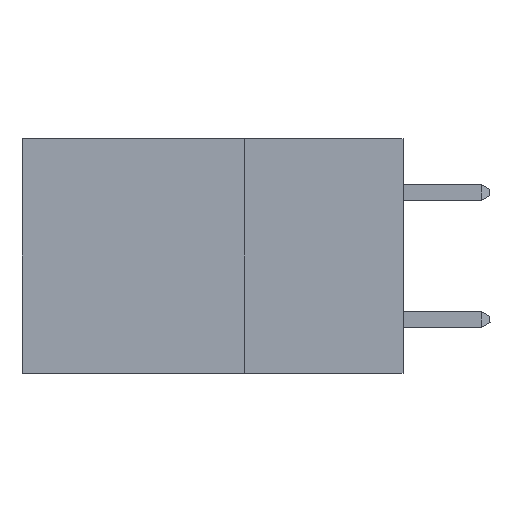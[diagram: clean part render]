
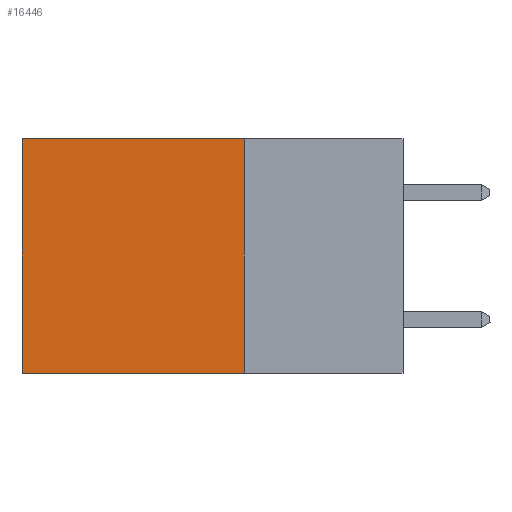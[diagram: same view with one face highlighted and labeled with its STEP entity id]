
A CAD part, left-side view. The second image highlights one B-rep face of the part: STEP entity #16446.
In plain terms, the highlighted planar face has unit normal (-1, 0, 0).
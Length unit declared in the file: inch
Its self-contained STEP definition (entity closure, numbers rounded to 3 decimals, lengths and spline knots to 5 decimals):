
#204 = CARTESIAN_POINT ( 'NONE',  ( 0.2875, 0.25, 0. ) ) ;
#271 = CARTESIAN_POINT ( 'NONE',  ( 0.2875, 0.25, 0. ) ) ;
#666 = VERTEX_POINT ( 'NONE', #271 ) ;
#736 = CARTESIAN_POINT ( 'NONE',  ( 0.2875, 0.25, 0. ) ) ;
#808 = DIRECTION ( 'NONE',  ( 0., 0., -1. ) ) ;
#1609 = ORIENTED_EDGE ( 'NONE', *, *, #37727, .T. ) ;
#2241 = ORIENTED_EDGE ( 'NONE', *, *, #41411, .T. ) ;
#2574 = LINE ( 'NONE', #204, #10060 ) ;
#3045 = AXIS2_PLACEMENT_3D ( 'NONE', #736, #20284, #32455 ) ;
#3133 = CARTESIAN_POINT ( 'NONE',  ( 0.2875, 0.25, 0. ) ) ;
#3269 = VECTOR ( 'NONE', #3585, 39.37008 ) ;
#3344 = VECTOR ( 'NONE', #16241, 39.37008 ) ;
#3539 = ORIENTED_EDGE ( 'NONE', *, *, #34445, .F. ) ;
#3585 = DIRECTION ( 'NONE',  ( 0., 1., 0. ) ) ;
#3780 = CARTESIAN_POINT ( 'NONE',  ( 0.2875, 0.6, 0. ) ) ;
#4105 = CARTESIAN_POINT ( 'NONE',  ( 0.2875, 0.6, 0. ) ) ;
#4383 = LINE ( 'NONE', #3133, #3344 ) ;
#9433 = VERTEX_POINT ( 'NONE', #32327 ) ;
#10060 = VECTOR ( 'NONE', #15874, 39.37008 ) ;
#15874 = DIRECTION ( 'NONE',  ( 0., 1., 0. ) ) ;
#16241 = DIRECTION ( 'NONE',  ( 0., 0., -1. ) ) ;
#16446 = ADVANCED_FACE ( 'NONE', ( #30501 ), #29390, .F. ) ;
#17302 = CARTESIAN_POINT ( 'NONE',  ( 0.2875, 0.6, -0.37 ) ) ;
#19489 = CARTESIAN_POINT ( 'NONE',  ( 0.2875, 0.25, -0.37 ) ) ;
#20284 = DIRECTION ( 'NONE',  ( 1., 0., 0. ) ) ;
#21241 = LINE ( 'NONE', #19489, #3269 ) ;
#24358 = VERTEX_POINT ( 'NONE', #4105 ) ;
#24741 = EDGE_LOOP ( 'NONE', ( #2241, #26404, #3539, #1609 ) ) ;
#26287 = VERTEX_POINT ( 'NONE', #17302 ) ;
#26404 = ORIENTED_EDGE ( 'NONE', *, *, #33804, .F. ) ;
#29390 = PLANE ( 'NONE',  #3045 ) ;
#30501 = FACE_OUTER_BOUND ( 'NONE', #24741, .T. ) ;
#32327 = CARTESIAN_POINT ( 'NONE',  ( 0.2875, 0.25, -0.37 ) ) ;
#32455 = DIRECTION ( 'NONE',  ( 0., 0., -1. ) ) ;
#33804 = EDGE_CURVE ( 'NONE', #9433, #26287, #21241, .T. ) ;
#34445 = EDGE_CURVE ( 'NONE', #666, #9433, #4383, .T. ) ;
#36208 = VECTOR ( 'NONE', #808, 39.37008 ) ;
#37727 = EDGE_CURVE ( 'NONE', #666, #24358, #2574, .T. ) ;
#38221 = LINE ( 'NONE', #3780, #36208 ) ;
#41411 = EDGE_CURVE ( 'NONE', #24358, #26287, #38221, .T. ) ;
